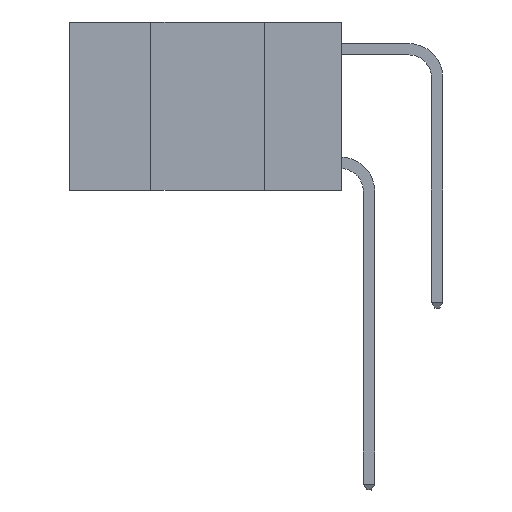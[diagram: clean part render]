
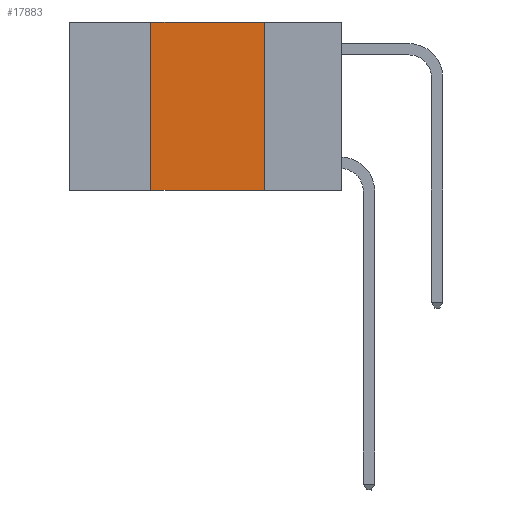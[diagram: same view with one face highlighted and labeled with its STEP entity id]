
A CAD part, left-side view. The second image highlights one B-rep face of the part: STEP entity #17883.
In plain terms, the highlighted planar face has unit normal (-1, 0, 0).
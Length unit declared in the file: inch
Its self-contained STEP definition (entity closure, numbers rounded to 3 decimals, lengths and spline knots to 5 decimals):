
#246 = LINE ( 'NONE', #24153, #736 ) ;
#736 = VECTOR ( 'NONE', #16515, 39.37008 ) ;
#1170 = DIRECTION ( 'NONE',  ( 0., 0., -1. ) ) ;
#2022 = CARTESIAN_POINT ( 'NONE',  ( 0., 0.42, 0. ) ) ;
#2089 = CARTESIAN_POINT ( 'NONE',  ( 0., 0.17, -0.37 ) ) ;
#2881 = VECTOR ( 'NONE', #12429, 39.37008 ) ;
#3740 = CARTESIAN_POINT ( 'NONE',  ( 0., 0.6, -0.37 ) ) ;
#3915 = LINE ( 'NONE', #3740, #27323 ) ;
#4725 = CARTESIAN_POINT ( 'NONE',  ( 0., 0.42, 0. ) ) ;
#5223 = AXIS2_PLACEMENT_3D ( 'NONE', #32676, #8928, #1170 ) ;
#7486 = VERTEX_POINT ( 'NONE', #4725 ) ;
#7544 = CARTESIAN_POINT ( 'NONE',  ( 0., 0.42, -0.37 ) ) ;
#8839 = ORIENTED_EDGE ( 'NONE', *, *, #17837, .T. ) ;
#8921 = EDGE_CURVE ( 'NONE', #29352, #17126, #246, .T. ) ;
#8928 = DIRECTION ( 'NONE',  ( 1., 0., 0. ) ) ;
#9908 = EDGE_CURVE ( 'NONE', #7486, #29352, #16268, .T. ) ;
#10117 = EDGE_CURVE ( 'NONE', #10377, #7486, #17633, .T. ) ;
#10377 = VERTEX_POINT ( 'NONE', #7544 ) ;
#10529 = CARTESIAN_POINT ( 'NONE',  ( 0., 0.6, 0. ) ) ;
#12410 = ORIENTED_EDGE ( 'NONE', *, *, #9908, .F. ) ;
#12429 = DIRECTION ( 'NONE',  ( 0., 0., 1. ) ) ;
#16063 = ORIENTED_EDGE ( 'NONE', *, *, #10117, .F. ) ;
#16268 = LINE ( 'NONE', #10529, #16733 ) ;
#16515 = DIRECTION ( 'NONE',  ( 0., 0., -1. ) ) ;
#16733 = VECTOR ( 'NONE', #16944, 39.37008 ) ;
#16944 = DIRECTION ( 'NONE',  ( 0., -1., 0. ) ) ;
#17126 = VERTEX_POINT ( 'NONE', #2089 ) ;
#17152 = EDGE_LOOP ( 'NONE', ( #33720, #12410, #16063, #8839 ) ) ;
#17633 = LINE ( 'NONE', #2022, #2881 ) ;
#17837 = EDGE_CURVE ( 'NONE', #10377, #17126, #3915, .T. ) ;
#17883 = ADVANCED_FACE ( 'NONE', ( #24903 ), #19536, .F. ) ;
#19536 = PLANE ( 'NONE',  #5223 ) ;
#21788 = DIRECTION ( 'NONE',  ( 0., -1., 0. ) ) ;
#23318 = CARTESIAN_POINT ( 'NONE',  ( 0., 0.17, 0. ) ) ;
#24153 = CARTESIAN_POINT ( 'NONE',  ( 0., 0.17, 0. ) ) ;
#24903 = FACE_OUTER_BOUND ( 'NONE', #17152, .T. ) ;
#27323 = VECTOR ( 'NONE', #21788, 39.37008 ) ;
#29352 = VERTEX_POINT ( 'NONE', #23318 ) ;
#32676 = CARTESIAN_POINT ( 'NONE',  ( 0., 0.6, 0. ) ) ;
#33720 = ORIENTED_EDGE ( 'NONE', *, *, #8921, .F. ) ;
